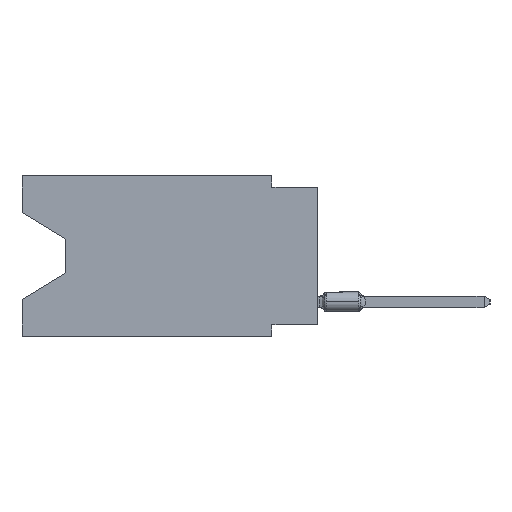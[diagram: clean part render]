
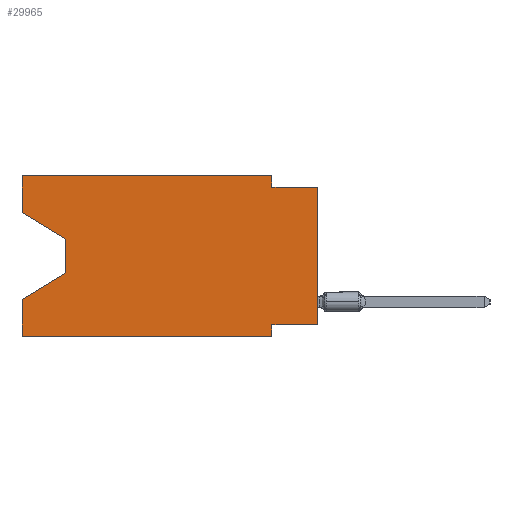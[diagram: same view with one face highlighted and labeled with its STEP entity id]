
A CAD part, left-side view. The second image highlights one B-rep face of the part: STEP entity #29965.
In plain terms, the highlighted planar face has unit normal (-1, 0, 0).
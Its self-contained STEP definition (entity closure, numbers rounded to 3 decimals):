
#276 = CARTESIAN_POINT ( 'NONE',  ( 0., 2.54, -8.89 ) ) ;
#874 = EDGE_CURVE ( 'NONE', #35442, #1798, #21957, .T. ) ;
#994 = EDGE_CURVE ( 'NONE', #8750, #24012, #15071, .T. ) ;
#1689 = ORIENTED_EDGE ( 'NONE', *, *, #13779, .F. ) ;
#1798 = VERTEX_POINT ( 'NONE', #10185 ) ;
#2129 = EDGE_CURVE ( 'NONE', #39465, #35442, #29219, .T. ) ;
#2738 = ORIENTED_EDGE ( 'NONE', *, *, #4248, .T. ) ;
#3540 = VECTOR ( 'NONE', #28561, 1000. ) ;
#4012 = LINE ( 'NONE', #7041, #3540 ) ;
#4248 = EDGE_CURVE ( 'NONE', #26342, #13266, #30492, .T. ) ;
#4618 = DIRECTION ( 'NONE',  ( 0., 0., 1. ) ) ;
#4791 = CARTESIAN_POINT ( 'NONE',  ( 0., 0., -0.635 ) ) ;
#5236 = LINE ( 'NONE', #35786, #17687 ) ;
#5255 = VECTOR ( 'NONE', #39584, 1000. ) ;
#5288 = LINE ( 'NONE', #8306, #27505 ) ;
#5339 = EDGE_CURVE ( 'NONE', #26342, #1798, #30019, .T. ) ;
#5468 = VERTEX_POINT ( 'NONE', #6256 ) ;
#6256 = CARTESIAN_POINT ( 'NONE',  ( 0., 0., -8.255 ) ) ;
#6560 = VERTEX_POINT ( 'NONE', #10455 ) ;
#7041 = CARTESIAN_POINT ( 'NONE',  ( 0., 0., -8.255 ) ) ;
#7348 = PLANE ( 'NONE',  #32476 ) ;
#8247 = DIRECTION ( 'NONE',  ( 0., -0.855, -0.519 ) ) ;
#8306 = CARTESIAN_POINT ( 'NONE',  ( 0., 0., 0. ) ) ;
#8452 = ORIENTED_EDGE ( 'NONE', *, *, #874, .T. ) ;
#8750 = VERTEX_POINT ( 'NONE', #28570 ) ;
#8961 = DIRECTION ( 'NONE',  ( 0., -1., 0. ) ) ;
#9551 = EDGE_CURVE ( 'NONE', #24012, #21680, #35814, .T. ) ;
#9630 = VECTOR ( 'NONE', #26308, 1000. ) ;
#9673 = CARTESIAN_POINT ( 'NONE',  ( 0., 13.97, -5.385 ) ) ;
#10185 = CARTESIAN_POINT ( 'NONE',  ( 0., 16.383, -6.852 ) ) ;
#10430 = ORIENTED_EDGE ( 'NONE', *, *, #994, .F. ) ;
#10455 = CARTESIAN_POINT ( 'NONE',  ( 0., 16.383, 0. ) ) ;
#10594 = ORIENTED_EDGE ( 'NONE', *, *, #9551, .F. ) ;
#11256 = CARTESIAN_POINT ( 'NONE',  ( 0., 16.383, -2.038 ) ) ;
#11276 = VERTEX_POINT ( 'NONE', #36011 ) ;
#11292 = CARTESIAN_POINT ( 'NONE',  ( 0., 0., -0.635 ) ) ;
#11900 = ORIENTED_EDGE ( 'NONE', *, *, #24330, .F. ) ;
#13266 = VERTEX_POINT ( 'NONE', #276 ) ;
#13539 = ORIENTED_EDGE ( 'NONE', *, *, #36071, .F. ) ;
#13779 = EDGE_CURVE ( 'NONE', #5468, #11276, #4012, .T. ) ;
#14003 = FACE_OUTER_BOUND ( 'NONE', #30722, .T. ) ;
#14886 = CARTESIAN_POINT ( 'NONE',  ( 0., 2.54, 0. ) ) ;
#15071 = LINE ( 'NONE', #14886, #5255 ) ;
#15224 = DIRECTION ( 'NONE',  ( 0., -1., 0. ) ) ;
#16020 = ORIENTED_EDGE ( 'NONE', *, *, #29162, .F. ) ;
#16561 = CARTESIAN_POINT ( 'NONE',  ( 0., 13.97, -3.505 ) ) ;
#16631 = DIRECTION ( 'NONE',  ( 0., 0., -1. ) ) ;
#17064 = ORIENTED_EDGE ( 'NONE', *, *, #18420, .T. ) ;
#17687 = VECTOR ( 'NONE', #4618, 1000. ) ;
#18341 = CARTESIAN_POINT ( 'NONE',  ( 0., 16.383, 0. ) ) ;
#18420 = EDGE_CURVE ( 'NONE', #5468, #21680, #5288, .T. ) ;
#18915 = CARTESIAN_POINT ( 'NONE',  ( 0., 13.97, -5.385 ) ) ;
#19281 = CARTESIAN_POINT ( 'NONE',  ( 0., 2.54, -0.635 ) ) ;
#19527 = DIRECTION ( 'NONE',  ( 0., 0.855, -0.519 ) ) ;
#19637 = CARTESIAN_POINT ( 'NONE',  ( 0., 16.383, 0. ) ) ;
#20773 = DIRECTION ( 'NONE',  ( 0., 0., 1. ) ) ;
#21680 = VERTEX_POINT ( 'NONE', #4791 ) ;
#21957 = LINE ( 'NONE', #9673, #25829 ) ;
#23000 = CARTESIAN_POINT ( 'NONE',  ( 0., 13.97, -3.505 ) ) ;
#23126 = VECTOR ( 'NONE', #15224, 1000. ) ;
#24012 = VERTEX_POINT ( 'NONE', #19281 ) ;
#24330 = EDGE_CURVE ( 'NONE', #6560, #8750, #33494, .T. ) ;
#25717 = LINE ( 'NONE', #29306, #9630 ) ;
#25829 = VECTOR ( 'NONE', #19527, 1000. ) ;
#26308 = DIRECTION ( 'NONE',  ( 0., 0., -1. ) ) ;
#26342 = VERTEX_POINT ( 'NONE', #34411 ) ;
#27505 = VECTOR ( 'NONE', #39658, 1000. ) ;
#27881 = CARTESIAN_POINT ( 'NONE',  ( 0., 16.383, -8.89 ) ) ;
#28561 = DIRECTION ( 'NONE',  ( 0., 1., 0. ) ) ;
#28570 = CARTESIAN_POINT ( 'NONE',  ( 0., 2.54, 0. ) ) ;
#29162 = EDGE_CURVE ( 'NONE', #36113, #6560, #5236, .T. ) ;
#29212 = EDGE_CURVE ( 'NONE', #36113, #39465, #38800, .T. ) ;
#29219 = LINE ( 'NONE', #23000, #32342 ) ;
#29306 = CARTESIAN_POINT ( 'NONE',  ( 0., 2.54, -8.89 ) ) ;
#29965 = ADVANCED_FACE ( 'NONE', ( #14003 ), #7348, .F. ) ;
#30019 = LINE ( 'NONE', #18341, #32463 ) ;
#30056 = ORIENTED_EDGE ( 'NONE', *, *, #29212, .T. ) ;
#30492 = LINE ( 'NONE', #27881, #23126 ) ;
#30722 = EDGE_LOOP ( 'NONE', ( #30056, #37131, #8452, #37015, #2738, #13539, #1689, #17064, #10594, #10430, #11900, #16020 ) ) ;
#31887 = DIRECTION ( 'NONE',  ( 1., 0., 0. ) ) ;
#32342 = VECTOR ( 'NONE', #38453, 1000. ) ;
#32463 = VECTOR ( 'NONE', #20773, 1000. ) ;
#32476 = AXIS2_PLACEMENT_3D ( 'NONE', #19637, #31887, #16631 ) ;
#33210 = DIRECTION ( 'NONE',  ( 0., -1., 0. ) ) ;
#33494 = LINE ( 'NONE', #36294, #35308 ) ;
#34339 = VECTOR ( 'NONE', #8247, 1000. ) ;
#34411 = CARTESIAN_POINT ( 'NONE',  ( 0., 16.383, -8.89 ) ) ;
#35308 = VECTOR ( 'NONE', #8961, 1000. ) ;
#35442 = VERTEX_POINT ( 'NONE', #18915 ) ;
#35715 = CARTESIAN_POINT ( 'NONE',  ( 0., 16.383, -2.038 ) ) ;
#35786 = CARTESIAN_POINT ( 'NONE',  ( 0., 16.383, 0. ) ) ;
#35814 = LINE ( 'NONE', #11292, #35974 ) ;
#35974 = VECTOR ( 'NONE', #33210, 1000. ) ;
#36011 = CARTESIAN_POINT ( 'NONE',  ( 0., 2.54, -8.255 ) ) ;
#36071 = EDGE_CURVE ( 'NONE', #11276, #13266, #25717, .T. ) ;
#36113 = VERTEX_POINT ( 'NONE', #35715 ) ;
#36294 = CARTESIAN_POINT ( 'NONE',  ( 0., 16.383, 0. ) ) ;
#37015 = ORIENTED_EDGE ( 'NONE', *, *, #5339, .F. ) ;
#37131 = ORIENTED_EDGE ( 'NONE', *, *, #2129, .T. ) ;
#38453 = DIRECTION ( 'NONE',  ( 0., 0., -1. ) ) ;
#38800 = LINE ( 'NONE', #11256, #34339 ) ;
#39465 = VERTEX_POINT ( 'NONE', #16561 ) ;
#39584 = DIRECTION ( 'NONE',  ( 0., 0., -1. ) ) ;
#39658 = DIRECTION ( 'NONE',  ( 0., 0., 1. ) ) ;
